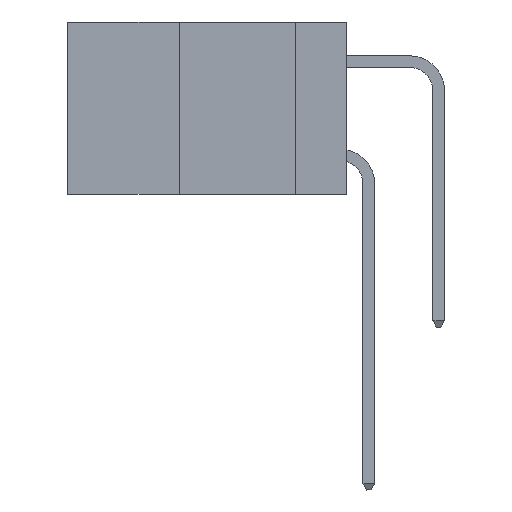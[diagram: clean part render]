
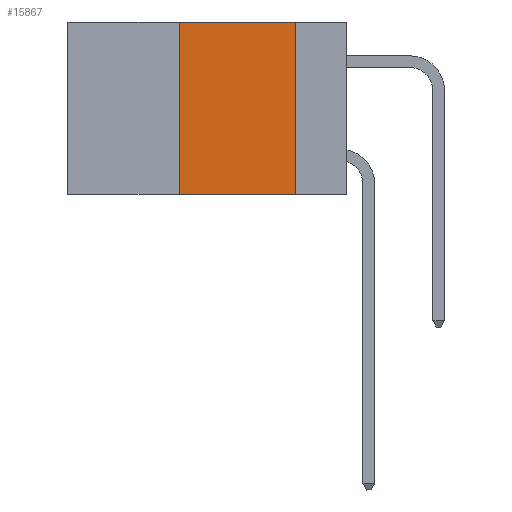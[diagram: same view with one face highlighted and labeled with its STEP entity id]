
A CAD part, left-side view. The second image highlights one B-rep face of the part: STEP entity #15867.
In plain terms, the highlighted planar face has unit normal (-1, 0, 0).
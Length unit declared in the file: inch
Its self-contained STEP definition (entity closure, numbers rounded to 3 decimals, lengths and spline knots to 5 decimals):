
#286 = LINE ( 'NONE', #666, #14229 ) ;
#541 = DIRECTION ( 'NONE',  ( 0., -1., 0. ) ) ;
#666 = CARTESIAN_POINT ( 'NONE',  ( 0., 0.11, 0. ) ) ;
#1612 = VERTEX_POINT ( 'NONE', #15501 ) ;
#2620 = EDGE_CURVE ( 'NONE', #1612, #10920, #5235, .T. ) ;
#3864 = DIRECTION ( 'NONE',  ( 0., 0., -1. ) ) ;
#3911 = VECTOR ( 'NONE', #5043, 39.37008 ) ;
#4487 = CARTESIAN_POINT ( 'NONE',  ( 0., 0.11, -0.37 ) ) ;
#5043 = DIRECTION ( 'NONE',  ( 0., 0., 1. ) ) ;
#5197 = EDGE_CURVE ( 'NONE', #14413, #7220, #286, .T. ) ;
#5235 = LINE ( 'NONE', #16094, #3911 ) ;
#5385 = PLANE ( 'NONE',  #15926 ) ;
#5951 = EDGE_LOOP ( 'NONE', ( #17741, #12301, #11485, #8106 ) ) ;
#6807 = VECTOR ( 'NONE', #541, 39.37008 ) ;
#7168 = CARTESIAN_POINT ( 'NONE',  ( 0., 0.6, 0. ) ) ;
#7220 = VERTEX_POINT ( 'NONE', #4487 ) ;
#7355 = FACE_OUTER_BOUND ( 'NONE', #5951, .T. ) ;
#8106 = ORIENTED_EDGE ( 'NONE', *, *, #12568, .T. ) ;
#8575 = LINE ( 'NONE', #10303, #17581 ) ;
#9074 = DIRECTION ( 'NONE',  ( 0., 0., -1. ) ) ;
#9207 = LINE ( 'NONE', #7168, #6807 ) ;
#10303 = CARTESIAN_POINT ( 'NONE',  ( 0., 0.6, -0.37 ) ) ;
#10920 = VERTEX_POINT ( 'NONE', #15404 ) ;
#11485 = ORIENTED_EDGE ( 'NONE', *, *, #2620, .F. ) ;
#12263 = CARTESIAN_POINT ( 'NONE',  ( 0., 0.6, 0. ) ) ;
#12301 = ORIENTED_EDGE ( 'NONE', *, *, #12907, .F. ) ;
#12568 = EDGE_CURVE ( 'NONE', #1612, #7220, #8575, .T. ) ;
#12907 = EDGE_CURVE ( 'NONE', #10920, #14413, #9207, .T. ) ;
#13259 = CARTESIAN_POINT ( 'NONE',  ( 0., 0.11, 0. ) ) ;
#14229 = VECTOR ( 'NONE', #9074, 39.37008 ) ;
#14413 = VERTEX_POINT ( 'NONE', #13259 ) ;
#14510 = DIRECTION ( 'NONE',  ( 0., -1., 0. ) ) ;
#15404 = CARTESIAN_POINT ( 'NONE',  ( 0., 0.36, 0. ) ) ;
#15501 = CARTESIAN_POINT ( 'NONE',  ( 0., 0.36, -0.37 ) ) ;
#15867 = ADVANCED_FACE ( 'NONE', ( #7355 ), #5385, .F. ) ;
#15926 = AXIS2_PLACEMENT_3D ( 'NONE', #12263, #16476, #3864 ) ;
#16094 = CARTESIAN_POINT ( 'NONE',  ( 0., 0.36, 0. ) ) ;
#16476 = DIRECTION ( 'NONE',  ( 1., 0., 0. ) ) ;
#17581 = VECTOR ( 'NONE', #14510, 39.37008 ) ;
#17741 = ORIENTED_EDGE ( 'NONE', *, *, #5197, .F. ) ;
